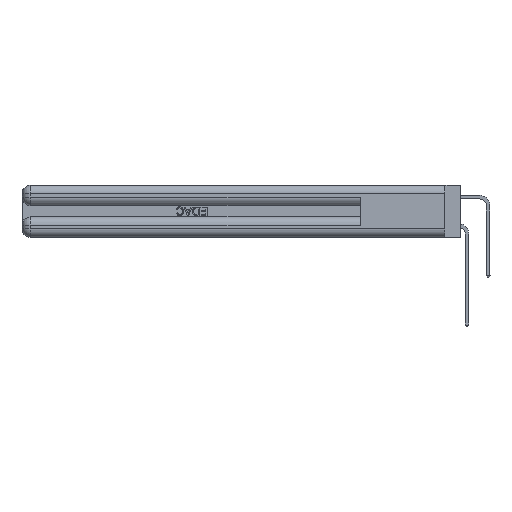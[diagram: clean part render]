
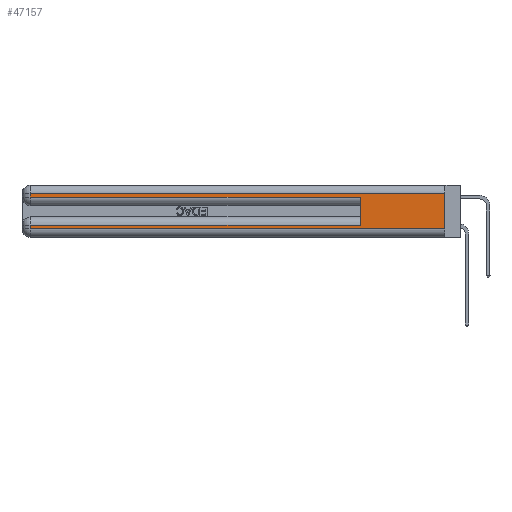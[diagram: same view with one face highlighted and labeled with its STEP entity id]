
A CAD part, left-side view. The second image highlights one B-rep face of the part: STEP entity #47157.
In plain terms, the highlighted planar face has unit normal (-1, 0, 0).
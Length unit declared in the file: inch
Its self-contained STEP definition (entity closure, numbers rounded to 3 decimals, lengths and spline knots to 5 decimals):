
#1500 = PLANE ( 'NONE',  #1713 ) ;
#1543 = CARTESIAN_POINT ( 'NONE',  ( 0., 2.94, 0.37 ) ) ;
#1713 = AXIS2_PLACEMENT_3D ( 'NONE', #42521, #27727, #5291 ) ;
#1946 = VERTEX_POINT ( 'NONE', #32302 ) ;
#1972 = ORIENTED_EDGE ( 'NONE', *, *, #18273, .T. ) ;
#2661 = VECTOR ( 'NONE', #41861, 39.37008 ) ;
#3818 = CARTESIAN_POINT ( 'NONE',  ( 0., 0.6, 0.145 ) ) ;
#4441 = VECTOR ( 'NONE', #35075, 39.37008 ) ;
#4763 = EDGE_CURVE ( 'NONE', #40013, #1946, #43219, .T. ) ;
#4942 = VERTEX_POINT ( 'NONE', #36758 ) ;
#5291 = DIRECTION ( 'NONE',  ( 0., 0., -1. ) ) ;
#5719 = CARTESIAN_POINT ( 'NONE',  ( 0., 2.94, 0.37 ) ) ;
#5730 = VECTOR ( 'NONE', #45327, 39.37008 ) ;
#5891 = CARTESIAN_POINT ( 'NONE',  ( 0., 0., 0.085 ) ) ;
#6154 = CARTESIAN_POINT ( 'NONE',  ( 0., 0.6, 0.085 ) ) ;
#6656 = VECTOR ( 'NONE', #46787, 39.37008 ) ;
#7294 = EDGE_CURVE ( 'NONE', #12255, #46509, #38867, .T. ) ;
#9389 = CARTESIAN_POINT ( 'NONE',  ( 0., 0.6, 0.285 ) ) ;
#9636 = DIRECTION ( 'NONE',  ( 0., 0., -1. ) ) ;
#10368 = VERTEX_POINT ( 'NONE', #29238 ) ;
#12255 = VERTEX_POINT ( 'NONE', #43214 ) ;
#12661 = LINE ( 'NONE', #15781, #2661 ) ;
#14045 = EDGE_CURVE ( 'NONE', #10368, #12255, #24361, .T. ) ;
#15781 = CARTESIAN_POINT ( 'NONE',  ( 0., 0., 0.31 ) ) ;
#16469 = VERTEX_POINT ( 'NONE', #34353 ) ;
#17174 = LINE ( 'NONE', #3818, #37034 ) ;
#18273 = EDGE_CURVE ( 'NONE', #1946, #4942, #41272, .T. ) ;
#19031 = VECTOR ( 'NONE', #42673, 39.37008 ) ;
#19263 = CARTESIAN_POINT ( 'NONE',  ( 0., 0., 0.37 ) ) ;
#20308 = CARTESIAN_POINT ( 'NONE',  ( 0., 0., 0.31 ) ) ;
#20378 = ORIENTED_EDGE ( 'NONE', *, *, #4763, .T. ) ;
#22199 = VECTOR ( 'NONE', #24535, 39.37008 ) ;
#23791 = ORIENTED_EDGE ( 'NONE', *, *, #38271, .F. ) ;
#24361 = LINE ( 'NONE', #1543, #4441 ) ;
#24455 = LINE ( 'NONE', #19263, #5730 ) ;
#24535 = DIRECTION ( 'NONE',  ( 0., 1., 0. ) ) ;
#24705 = EDGE_CURVE ( 'NONE', #30003, #16469, #24455, .T. ) ;
#26274 = DIRECTION ( 'NONE',  ( 0., 0., 1. ) ) ;
#26583 = EDGE_CURVE ( 'NONE', #30003, #10368, #12661, .T. ) ;
#27727 = DIRECTION ( 'NONE',  ( 1., 0., 0. ) ) ;
#27767 = ORIENTED_EDGE ( 'NONE', *, *, #26583, .T. ) ;
#28256 = CARTESIAN_POINT ( 'NONE',  ( 0., 0., 0.06 ) ) ;
#29238 = CARTESIAN_POINT ( 'NONE',  ( 0., 2.94, 0.31 ) ) ;
#29810 = FACE_OUTER_BOUND ( 'NONE', #38120, .T. ) ;
#30003 = VERTEX_POINT ( 'NONE', #20308 ) ;
#31362 = VECTOR ( 'NONE', #9636, 39.37008 ) ;
#31445 = CARTESIAN_POINT ( 'NONE',  ( 0., 0., 0.285 ) ) ;
#32302 = CARTESIAN_POINT ( 'NONE',  ( 0., 2.94, 0.085 ) ) ;
#33286 = EDGE_CURVE ( 'NONE', #4942, #16469, #45192, .T. ) ;
#33781 = ORIENTED_EDGE ( 'NONE', *, *, #14045, .T. ) ;
#34353 = CARTESIAN_POINT ( 'NONE',  ( 0., 0., 0.06 ) ) ;
#34414 = ORIENTED_EDGE ( 'NONE', *, *, #7294, .T. ) ;
#35075 = DIRECTION ( 'NONE',  ( 0., 0., -1. ) ) ;
#36758 = CARTESIAN_POINT ( 'NONE',  ( 0., 2.94, 0.06 ) ) ;
#37034 = VECTOR ( 'NONE', #26274, 39.37008 ) ;
#38120 = EDGE_LOOP ( 'NONE', ( #45177, #27767, #33781, #34414, #23791, #20378, #1972, #44765 ) ) ;
#38271 = EDGE_CURVE ( 'NONE', #40013, #46509, #17174, .T. ) ;
#38867 = LINE ( 'NONE', #31445, #19031 ) ;
#40013 = VERTEX_POINT ( 'NONE', #6154 ) ;
#41272 = LINE ( 'NONE', #5719, #31362 ) ;
#41861 = DIRECTION ( 'NONE',  ( 0., 1., 0. ) ) ;
#42521 = CARTESIAN_POINT ( 'NONE',  ( 0., 0., 0.37 ) ) ;
#42673 = DIRECTION ( 'NONE',  ( 0., -1., 0. ) ) ;
#43214 = CARTESIAN_POINT ( 'NONE',  ( 0., 2.94, 0.285 ) ) ;
#43219 = LINE ( 'NONE', #5891, #22199 ) ;
#44765 = ORIENTED_EDGE ( 'NONE', *, *, #33286, .T. ) ;
#45177 = ORIENTED_EDGE ( 'NONE', *, *, #24705, .F. ) ;
#45192 = LINE ( 'NONE', #28256, #6656 ) ;
#45327 = DIRECTION ( 'NONE',  ( 0., 0., -1. ) ) ;
#46509 = VERTEX_POINT ( 'NONE', #9389 ) ;
#46787 = DIRECTION ( 'NONE',  ( 0., -1., 0. ) ) ;
#47157 = ADVANCED_FACE ( 'NONE', ( #29810 ), #1500, .F. ) ;
